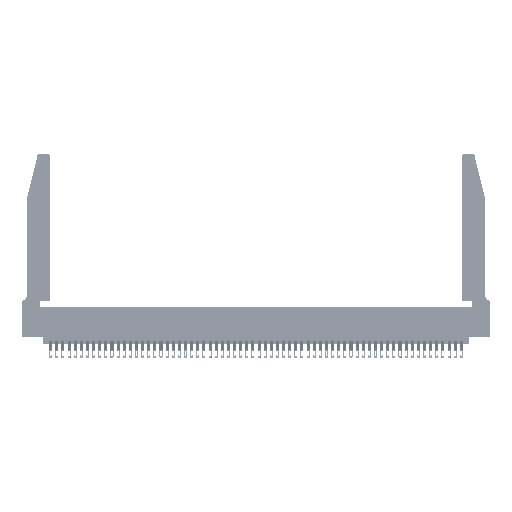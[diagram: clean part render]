
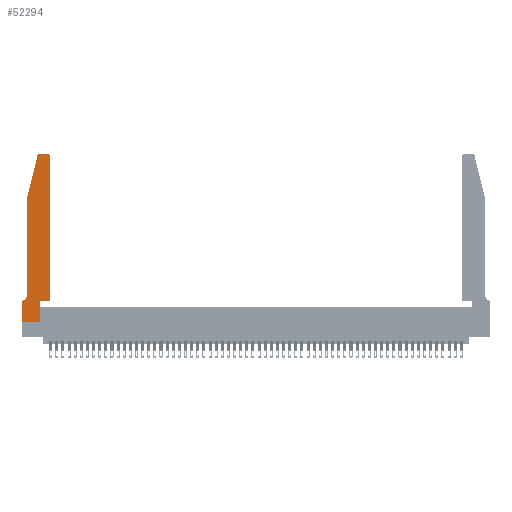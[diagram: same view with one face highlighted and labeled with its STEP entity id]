
A CAD part, top view. The second image highlights one B-rep face of the part: STEP entity #52294.
In plain terms, the highlighted planar face has unit normal (0, 0, 1).
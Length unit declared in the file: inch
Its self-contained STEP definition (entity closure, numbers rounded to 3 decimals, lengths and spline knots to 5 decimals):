
#64 = CIRCLE ( 'NONE', #11878, 0.03 ) ;
#900 = CARTESIAN_POINT ( 'NONE',  ( 0.0755, 2., 0.37 ) ) ;
#1463 = DIRECTION ( 'NONE',  ( 0., 0., 1. ) ) ;
#1492 = CARTESIAN_POINT ( 'NONE',  ( 0.0755, 0.35, 0.37 ) ) ;
#3284 = ORIENTED_EDGE ( 'NONE', *, *, #5526, .T. ) ;
#3362 = EDGE_CURVE ( 'NONE', #45933, #46333, #9663, .T. ) ;
#4050 = VERTEX_POINT ( 'NONE', #9122 ) ;
#4125 = CARTESIAN_POINT ( 'NONE',  ( 0.2865, 0.35, 0.37 ) ) ;
#4714 = CARTESIAN_POINT ( 'NONE',  ( 0., 0.35, 0.37 ) ) ;
#4750 = DIRECTION ( 'NONE',  ( -1., 0., 0. ) ) ;
#5526 = EDGE_CURVE ( 'NONE', #22037, #37679, #6425, .T. ) ;
#6066 = CARTESIAN_POINT ( 'NONE',  ( 0., 0.35, 0.37 ) ) ;
#6425 = LINE ( 'NONE', #1492, #34390 ) ;
#6461 = CARTESIAN_POINT ( 'NONE',  ( 0.0755, 0.42, 0.37 ) ) ;
#7624 = ORIENTED_EDGE ( 'NONE', *, *, #45690, .T. ) ;
#7731 = DIRECTION ( 'NONE',  ( 1., 0., 0. ) ) ;
#8223 = LINE ( 'NONE', #41742, #48847 ) ;
#8769 = PLANE ( 'NONE',  #15259 ) ;
#9122 = CARTESIAN_POINT ( 'NONE',  ( 0.4505, 0.35, 0.37 ) ) ;
#9663 = LINE ( 'NONE', #31501, #18351 ) ;
#10495 = CARTESIAN_POINT ( 'NONE',  ( 0.284, 2.75, 0.37 ) ) ;
#10815 = DIRECTION ( 'NONE',  ( -1., 0., 0. ) ) ;
#11168 = ORIENTED_EDGE ( 'NONE', *, *, #20540, .T. ) ;
#11543 = VECTOR ( 'NONE', #34676, 39.37008 ) ;
#11878 = AXIS2_PLACEMENT_3D ( 'NONE', #22689, #1463, #39224 ) ;
#12442 = CIRCLE ( 'NONE', #14560, 0.07 ) ;
#12920 = CARTESIAN_POINT ( 'NONE',  ( 0.0055, 0.42, 0.37 ) ) ;
#13038 = LINE ( 'NONE', #14726, #24960 ) ;
#13258 = DIRECTION ( 'NONE',  ( 0., 0., 1. ) ) ;
#13662 = DIRECTION ( 'NONE',  ( 0., 1., 0. ) ) ;
#14550 = DIRECTION ( 'NONE',  ( 0., -1., 0. ) ) ;
#14560 = AXIS2_PLACEMENT_3D ( 'NONE', #12920, #34737, #4750 ) ;
#14726 = CARTESIAN_POINT ( 'NONE',  ( 0.0755, 2., 0.37 ) ) ;
#15068 = VECTOR ( 'NONE', #7731, 39.37008 ) ;
#15259 = AXIS2_PLACEMENT_3D ( 'NONE', #4714, #13258, #38596 ) ;
#15601 = VERTEX_POINT ( 'NONE', #50127 ) ;
#15663 = VERTEX_POINT ( 'NONE', #51228 ) ;
#15935 = ORIENTED_EDGE ( 'NONE', *, *, #3362, .T. ) ;
#16630 = ORIENTED_EDGE ( 'NONE', *, *, #32501, .T. ) ;
#18351 = VECTOR ( 'NONE', #10815, 39.37008 ) ;
#18920 = LINE ( 'NONE', #34495, #11543 ) ;
#19516 = EDGE_CURVE ( 'NONE', #28345, #4050, #44276, .T. ) ;
#19802 = VECTOR ( 'NONE', #13662, 39.37008 ) ;
#19876 = VERTEX_POINT ( 'NONE', #20052 ) ;
#20052 = CARTESIAN_POINT ( 'NONE',  ( 0.0755, 2., 0.37 ) ) ;
#20295 = CARTESIAN_POINT ( 'NONE',  ( 0., 0., 0.37 ) ) ;
#20540 = EDGE_CURVE ( 'NONE', #4050, #15601, #8223, .T. ) ;
#21509 = EDGE_CURVE ( 'NONE', #15663, #19876, #22860, .T. ) ;
#22037 = VERTEX_POINT ( 'NONE', #23707 ) ;
#22689 = CARTESIAN_POINT ( 'NONE',  ( 0.284, 2.72, 0.37 ) ) ;
#22860 = LINE ( 'NONE', #900, #38786 ) ;
#23707 = CARTESIAN_POINT ( 'NONE',  ( 0.0055, 0.35, 0.37 ) ) ;
#24534 = CIRCLE ( 'NONE', #50604, 0.03 ) ;
#24623 = VERTEX_POINT ( 'NONE', #6461 ) ;
#24638 = ORIENTED_EDGE ( 'NONE', *, *, #19516, .T. ) ;
#24960 = VECTOR ( 'NONE', #14550, 39.37008 ) ;
#25122 = LINE ( 'NONE', #26543, #19802 ) ;
#25215 = ORIENTED_EDGE ( 'NONE', *, *, #27159, .T. ) ;
#26543 = CARTESIAN_POINT ( 'NONE',  ( 0.2865, 0.35, 0.37 ) ) ;
#26610 = DIRECTION ( 'NONE',  ( -1., 0., 0. ) ) ;
#27019 = EDGE_CURVE ( 'NONE', #24623, #22037, #12442, .T. ) ;
#27159 = EDGE_CURVE ( 'NONE', #33748, #28345, #25122, .T. ) ;
#27285 = EDGE_LOOP ( 'NONE', ( #15935, #28809, #49779, #7624, #29764, #3284, #16630, #39870, #25215, #24638, #11168, #47175 ) ) ;
#28345 = VERTEX_POINT ( 'NONE', #4125 ) ;
#28784 = VERTEX_POINT ( 'NONE', #20295 ) ;
#28809 = ORIENTED_EDGE ( 'NONE', *, *, #48240, .T. ) ;
#28861 = CARTESIAN_POINT ( 'NONE',  ( 0.4205, 2.75, 0.37 ) ) ;
#28966 = CARTESIAN_POINT ( 'NONE',  ( 0., 0., 0.37 ) ) ;
#29764 = ORIENTED_EDGE ( 'NONE', *, *, #27019, .T. ) ;
#30295 = DIRECTION ( 'NONE',  ( -0.239, -0.971, 0. ) ) ;
#31501 = CARTESIAN_POINT ( 'NONE',  ( 0.2605, 2.75, 0.37 ) ) ;
#32501 = EDGE_CURVE ( 'NONE', #37679, #28784, #18920, .T. ) ;
#32957 = VECTOR ( 'NONE', #46638, 39.37008 ) ;
#33748 = VERTEX_POINT ( 'NONE', #47810 ) ;
#34390 = VECTOR ( 'NONE', #26610, 39.37008 ) ;
#34427 = LINE ( 'NONE', #28966, #15068 ) ;
#34495 = CARTESIAN_POINT ( 'NONE',  ( 0., 0., 0.37 ) ) ;
#34676 = DIRECTION ( 'NONE',  ( 0., -1., 0. ) ) ;
#34737 = DIRECTION ( 'NONE',  ( 0., 0., -1. ) ) ;
#37679 = VERTEX_POINT ( 'NONE', #6066 ) ;
#38596 = DIRECTION ( 'NONE',  ( 1., 0., 0. ) ) ;
#38786 = VECTOR ( 'NONE', #30295, 39.37008 ) ;
#39224 = DIRECTION ( 'NONE',  ( 1., 0., 0. ) ) ;
#39870 = ORIENTED_EDGE ( 'NONE', *, *, #44678, .T. ) ;
#41742 = CARTESIAN_POINT ( 'NONE',  ( 0.4505, 0.35, 0.37 ) ) ;
#42502 = CARTESIAN_POINT ( 'NONE',  ( 0.4205, 2.72, 0.37 ) ) ;
#43537 = EDGE_CURVE ( 'NONE', #15601, #45933, #24534, .T. ) ;
#44276 = LINE ( 'NONE', #50913, #32957 ) ;
#44678 = EDGE_CURVE ( 'NONE', #28784, #33748, #34427, .T. ) ;
#45444 = DIRECTION ( 'NONE',  ( 0., 1., 0. ) ) ;
#45690 = EDGE_CURVE ( 'NONE', #19876, #24623, #13038, .T. ) ;
#45933 = VERTEX_POINT ( 'NONE', #28861 ) ;
#46333 = VERTEX_POINT ( 'NONE', #10495 ) ;
#46638 = DIRECTION ( 'NONE',  ( 1., 0., 0. ) ) ;
#46745 = DIRECTION ( 'NONE',  ( 1., 0., 0. ) ) ;
#47175 = ORIENTED_EDGE ( 'NONE', *, *, #43537, .T. ) ;
#47809 = DIRECTION ( 'NONE',  ( 0., 0., 1. ) ) ;
#47810 = CARTESIAN_POINT ( 'NONE',  ( 0.2865, 0., 0.37 ) ) ;
#48240 = EDGE_CURVE ( 'NONE', #46333, #15663, #64, .T. ) ;
#48847 = VECTOR ( 'NONE', #45444, 39.37008 ) ;
#49779 = ORIENTED_EDGE ( 'NONE', *, *, #21509, .T. ) ;
#50127 = CARTESIAN_POINT ( 'NONE',  ( 0.4505, 2.72, 0.37 ) ) ;
#50604 = AXIS2_PLACEMENT_3D ( 'NONE', #42502, #47809, #46745 ) ;
#50913 = CARTESIAN_POINT ( 'NONE',  ( 0.4505, 0.35, 0.37 ) ) ;
#51228 = CARTESIAN_POINT ( 'NONE',  ( 0.25487, 2.72718, 0.37 ) ) ;
#52294 = ADVANCED_FACE ( 'NONE', ( #54910 ), #8769, .T. ) ;
#54910 = FACE_OUTER_BOUND ( 'NONE', #27285, .T. ) ;
